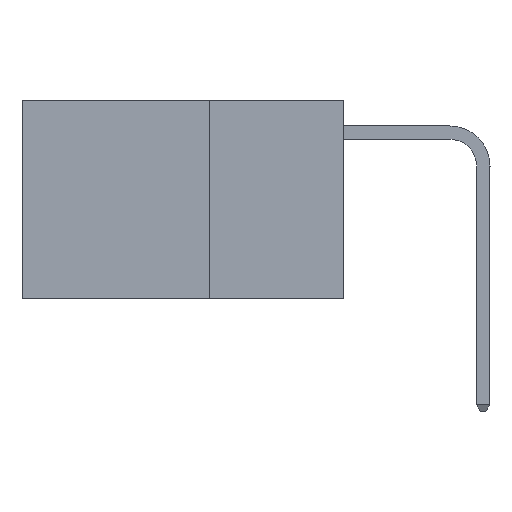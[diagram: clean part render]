
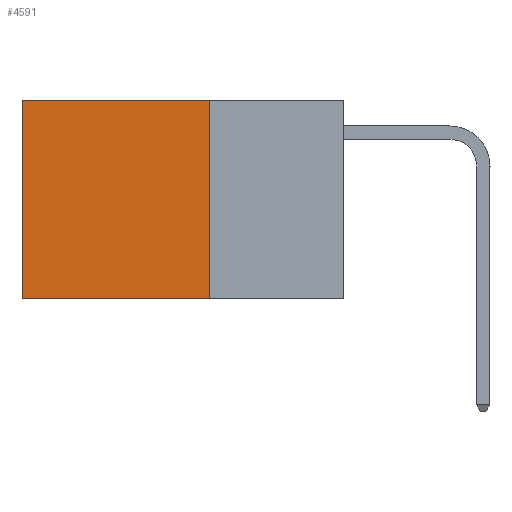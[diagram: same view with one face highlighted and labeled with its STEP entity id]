
A CAD part, left-side view. The second image highlights one B-rep face of the part: STEP entity #4591.
In plain terms, the highlighted planar face has unit normal (-1, 0, 0).
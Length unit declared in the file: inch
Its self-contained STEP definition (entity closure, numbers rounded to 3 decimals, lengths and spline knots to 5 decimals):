
#856 = EDGE_CURVE ( 'NONE', #13913, #12252, #11004, .T. ) ;
#983 = CARTESIAN_POINT ( 'NONE',  ( 0.2625, 0.25, 0. ) ) ;
#1278 = VECTOR ( 'NONE', #12725, 39.37008 ) ;
#2057 = AXIS2_PLACEMENT_3D ( 'NONE', #6230, #6128, #6097 ) ;
#2818 = ORIENTED_EDGE ( 'NONE', *, *, #3880, .F. ) ;
#3494 = DIRECTION ( 'NONE',  ( 0., 0., -1. ) ) ;
#3787 = DIRECTION ( 'NONE',  ( 0., 0., -1. ) ) ;
#3854 = CARTESIAN_POINT ( 'NONE',  ( 0.2625, 0.25, 0. ) ) ;
#3880 = EDGE_CURVE ( 'NONE', #13913, #13957, #10735, .T. ) ;
#4504 = ORIENTED_EDGE ( 'NONE', *, *, #6033, .T. ) ;
#4591 = ADVANCED_FACE ( 'NONE', ( #8478 ), #6388, .F. ) ;
#4842 = VECTOR ( 'NONE', #3787, 39.37008 ) ;
#5110 = VECTOR ( 'NONE', #5978, 39.37008 ) ;
#5978 = DIRECTION ( 'NONE',  ( 0., 1., 0. ) ) ;
#6033 = EDGE_CURVE ( 'NONE', #12252, #7323, #10686, .T. ) ;
#6097 = DIRECTION ( 'NONE',  ( 0., 0., -1. ) ) ;
#6128 = DIRECTION ( 'NONE',  ( 1., 0., 0. ) ) ;
#6214 = CARTESIAN_POINT ( 'NONE',  ( 0.2625, 0.25, -0.37 ) ) ;
#6230 = CARTESIAN_POINT ( 'NONE',  ( 0.2625, 0.25, 0. ) ) ;
#6388 = PLANE ( 'NONE',  #2057 ) ;
#6417 = ORIENTED_EDGE ( 'NONE', *, *, #856, .T. ) ;
#7323 = VERTEX_POINT ( 'NONE', #10323 ) ;
#7751 = VECTOR ( 'NONE', #3494, 39.37008 ) ;
#8478 = FACE_OUTER_BOUND ( 'NONE', #13699, .T. ) ;
#9813 = CARTESIAN_POINT ( 'NONE',  ( 0.2625, 0.25, 0. ) ) ;
#10129 = CARTESIAN_POINT ( 'NONE',  ( 0.2625, 0.6, 0. ) ) ;
#10323 = CARTESIAN_POINT ( 'NONE',  ( 0.2625, 0.6, -0.37 ) ) ;
#10640 = ORIENTED_EDGE ( 'NONE', *, *, #12374, .F. ) ;
#10686 = LINE ( 'NONE', #10129, #7751 ) ;
#10735 = LINE ( 'NONE', #3854, #4842 ) ;
#11004 = LINE ( 'NONE', #9813, #5110 ) ;
#12252 = VERTEX_POINT ( 'NONE', #13346 ) ;
#12374 = EDGE_CURVE ( 'NONE', #13957, #7323, #13410, .T. ) ;
#12725 = DIRECTION ( 'NONE',  ( 0., 1., 0. ) ) ;
#13246 = CARTESIAN_POINT ( 'NONE',  ( 0.2625, 0.25, -0.37 ) ) ;
#13346 = CARTESIAN_POINT ( 'NONE',  ( 0.2625, 0.6, 0. ) ) ;
#13410 = LINE ( 'NONE', #6214, #1278 ) ;
#13699 = EDGE_LOOP ( 'NONE', ( #4504, #10640, #2818, #6417 ) ) ;
#13913 = VERTEX_POINT ( 'NONE', #983 ) ;
#13957 = VERTEX_POINT ( 'NONE', #13246 ) ;
